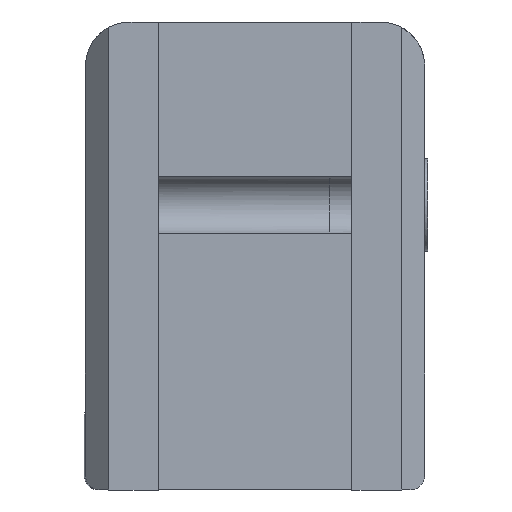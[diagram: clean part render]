
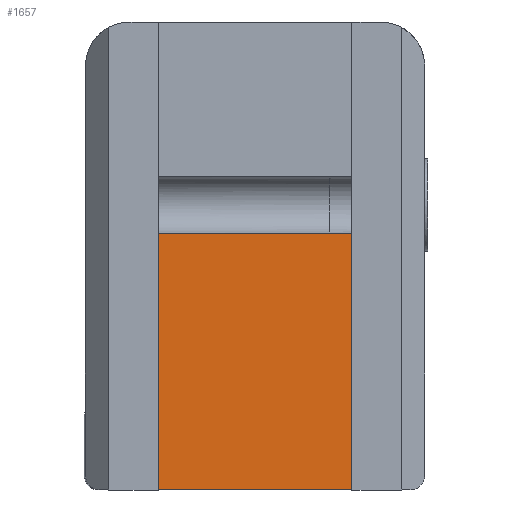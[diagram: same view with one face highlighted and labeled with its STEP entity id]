
A CAD part, front view. The second image highlights one B-rep face of the part: STEP entity #1657.
In plain terms, the highlighted planar face has unit normal (0, -1, 0).
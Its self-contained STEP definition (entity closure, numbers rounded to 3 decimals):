
#60=PLANE('',#1820);
#149=FACE_OUTER_BOUND('',#243,.T.);
#243=EDGE_LOOP('',(#1425,#1426,#1427,#1428,#1429,#1430));
#425=LINE('',#2760,#542);
#465=LINE('',#3454,#582);
#466=LINE('',#3456,#583);
#467=LINE('',#3458,#584);
#468=LINE('',#3460,#585);
#469=LINE('',#3461,#586);
#542=VECTOR('',#2032,10.);
#582=VECTOR('',#2218,10.);
#583=VECTOR('',#2219,10.);
#584=VECTOR('',#2220,10.);
#585=VECTOR('',#2221,10.);
#586=VECTOR('',#2222,10.);
#713=VERTEX_POINT('',#2757);
#714=VERTEX_POINT('',#2759);
#769=VERTEX_POINT('',#3453);
#770=VERTEX_POINT('',#3455);
#771=VERTEX_POINT('',#3457);
#772=VERTEX_POINT('',#3459);
#895=EDGE_CURVE('',#713,#714,#425,.T.);
#1002=EDGE_CURVE('',#713,#769,#465,.T.);
#1003=EDGE_CURVE('',#769,#770,#466,.T.);
#1004=EDGE_CURVE('',#770,#771,#467,.T.);
#1005=EDGE_CURVE('',#772,#771,#468,.T.);
#1006=EDGE_CURVE('',#714,#772,#469,.T.);
#1425=ORIENTED_EDGE('',*,*,#895,.F.);
#1426=ORIENTED_EDGE('',*,*,#1002,.T.);
#1427=ORIENTED_EDGE('',*,*,#1003,.T.);
#1428=ORIENTED_EDGE('',*,*,#1004,.T.);
#1429=ORIENTED_EDGE('',*,*,#1005,.F.);
#1430=ORIENTED_EDGE('',*,*,#1006,.F.);
#1657=ADVANCED_FACE('',(#149),#60,.F.);
#1820=AXIS2_PLACEMENT_3D('',#3452,#2216,#2217);
#2032=DIRECTION('',(-1.,0.,0.));
#2216=DIRECTION('center_axis',(0.,1.,0.));
#2217=DIRECTION('ref_axis',(-1.,0.,0.));
#2218=DIRECTION('',(0.,0.,1.));
#2219=DIRECTION('',(-1.,0.,0.));
#2220=DIRECTION('',(0.,0.,1.));
#2221=DIRECTION('',(1.,0.,0.));
#2222=DIRECTION('',(0.,0.,1.));
#2757=CARTESIAN_POINT('',(7.712,73.777,-58.601));
#2759=CARTESIAN_POINT('',(-8.848,73.777,-58.601));
#2760=CARTESIAN_POINT('',(-0.688,73.777,-58.601));
#3452=CARTESIAN_POINT('Origin',(7.472,73.777,-58.601));
#3453=CARTESIAN_POINT('',(7.712,73.776,-36.665));
#3454=CARTESIAN_POINT('',(7.712,73.776,-28.28));
#3455=CARTESIAN_POINT('',(5.82,73.776,-36.665));
#3456=CARTESIAN_POINT('',(14.202,73.776,-36.665));
#3457=CARTESIAN_POINT('',(5.82,73.776,-36.648));
#3458=CARTESIAN_POINT('',(5.82,73.777,-46.424));
#3459=CARTESIAN_POINT('',(-8.848,73.776,-36.648));
#3460=CARTESIAN_POINT('',(2.932,73.776,-36.648));
#3461=CARTESIAN_POINT('',(-8.848,73.776,-28.28));
